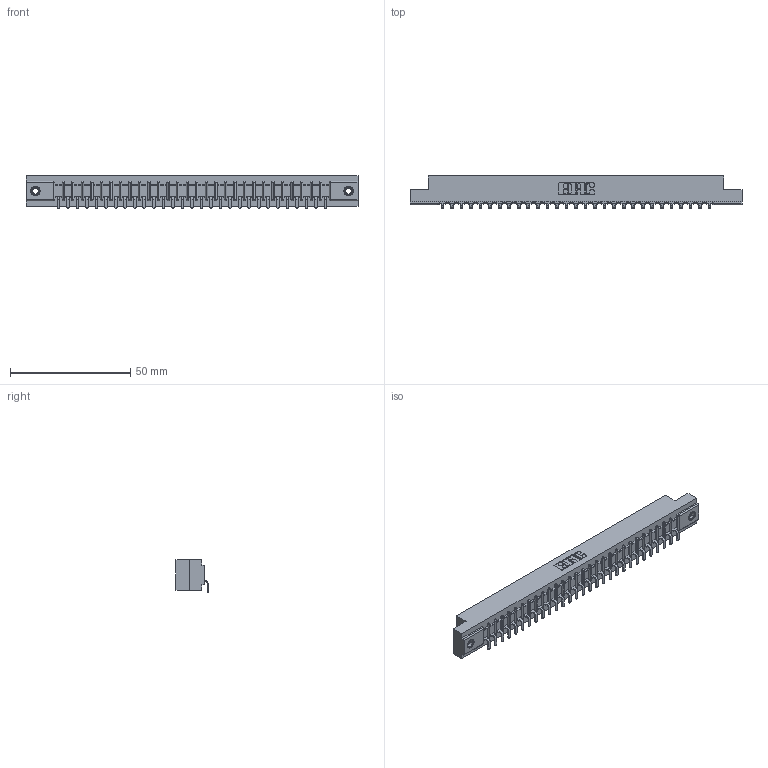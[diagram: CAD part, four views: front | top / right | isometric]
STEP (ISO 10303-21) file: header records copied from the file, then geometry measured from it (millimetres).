
FILE_DESCRIPTION (( 'STEP AP203' ), '1' );
FILE_NAME ('357-029-553-107.STEP', '2019-09-17T02:44:36', ( '' ), ( '' ), 'SwSTEP 2.0', 'SolidWorks 2016', '' );
FILE_SCHEMA (( 'CONFIG_CONTROL_DESIGN' ));
Length unit declared in the file: inch
Products named in the file (4): 307 Part_.156 Dia Mounting Holes; 307-290-002_553; 345-250-001_345-250-005-103; 357-029-553-107
Assembly tree (32 placements, depth 2):
  357-029-553-107
    307 Part_.156 Dia Mounting Holes
    307-290-002_553  x29
    345-250-001_345-250-005-103  x2
Bounding box: 137.92 x 13.32 x 13.5 mm (x, y, z)
Volume: 14648.8 mm3; surface area: 18162 mm2
Topology: 32 solids, 32 shells, 2470 faces, 7535 edges, 4934 vertices
Faces by surface type: plane 1465, cylinder 929, sphere 60, cone 12, torus 4
Entity records: 28503 total; most frequent: CARTESIAN_POINT 4787, ORIENTED_EDGE 4770, DIRECTION 4667, EDGE_CURVE 2385, LINE 1819, VECTOR 1819, VERTEX_POINT 1544, AXIS2_PLACEMENT_3D 1424
